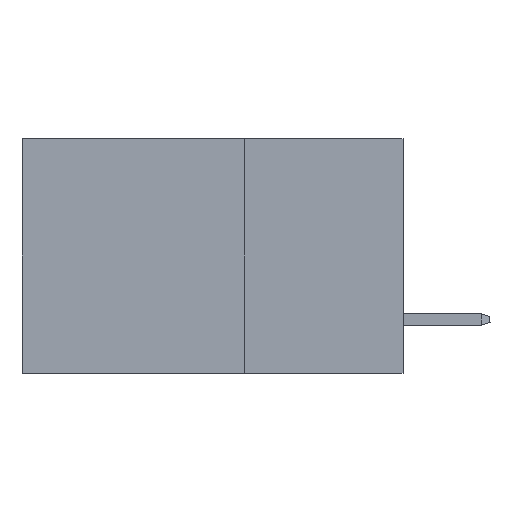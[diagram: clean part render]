
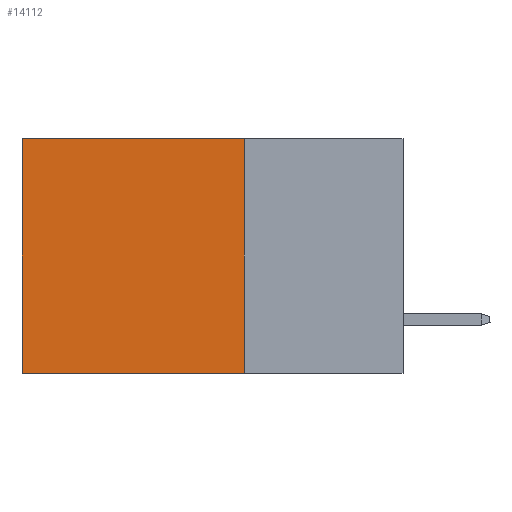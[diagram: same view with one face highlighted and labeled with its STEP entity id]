
A CAD part, left-side view. The second image highlights one B-rep face of the part: STEP entity #14112.
In plain terms, the highlighted planar face has unit normal (-1, 0, 0).
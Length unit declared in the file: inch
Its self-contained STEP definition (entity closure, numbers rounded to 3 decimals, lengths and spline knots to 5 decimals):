
#760 = CARTESIAN_POINT ( 'NONE',  ( 0.2875, 0.25, -0.37 ) ) ;
#1092 = DIRECTION ( 'NONE',  ( 1., 0., 0. ) ) ;
#1314 = CARTESIAN_POINT ( 'NONE',  ( 0.2875, 0.25, 0. ) ) ;
#2424 = VECTOR ( 'NONE', #29652, 39.37008 ) ;
#4251 = LINE ( 'NONE', #760, #14232 ) ;
#4681 = DIRECTION ( 'NONE',  ( 0., 0., -1. ) ) ;
#7620 = DIRECTION ( 'NONE',  ( 0., 0., -1. ) ) ;
#8201 = VERTEX_POINT ( 'NONE', #20159 ) ;
#8949 = ORIENTED_EDGE ( 'NONE', *, *, #25783, .T. ) ;
#11808 = CARTESIAN_POINT ( 'NONE',  ( 0.2875, 0.6, 0. ) ) ;
#12774 = CARTESIAN_POINT ( 'NONE',  ( 0.2875, 0.6, 0. ) ) ;
#12900 = EDGE_CURVE ( 'NONE', #28885, #45731, #36372, .T. ) ;
#14112 = ADVANCED_FACE ( 'NONE', ( #40319 ), #22231, .F. ) ;
#14232 = VECTOR ( 'NONE', #36275, 39.37008 ) ;
#15372 = VERTEX_POINT ( 'NONE', #40328 ) ;
#15742 = LINE ( 'NONE', #11808, #28760 ) ;
#15960 = EDGE_LOOP ( 'NONE', ( #8949, #40078, #38517, #32553 ) ) ;
#16264 = CARTESIAN_POINT ( 'NONE',  ( 0.2875, 0.25, 0. ) ) ;
#20159 = CARTESIAN_POINT ( 'NONE',  ( 0.2875, 0.25, -0.37 ) ) ;
#22231 = PLANE ( 'NONE',  #26239 ) ;
#25783 = EDGE_CURVE ( 'NONE', #45731, #15372, #15742, .T. ) ;
#26239 = AXIS2_PLACEMENT_3D ( 'NONE', #29213, #1092, #7620 ) ;
#28760 = VECTOR ( 'NONE', #44047, 39.37008 ) ;
#28885 = VERTEX_POINT ( 'NONE', #34883 ) ;
#29213 = CARTESIAN_POINT ( 'NONE',  ( 0.2875, 0.25, 0. ) ) ;
#29652 = DIRECTION ( 'NONE',  ( 0., 1., 0. ) ) ;
#31591 = EDGE_CURVE ( 'NONE', #8201, #15372, #4251, .T. ) ;
#32553 = ORIENTED_EDGE ( 'NONE', *, *, #12900, .T. ) ;
#33876 = LINE ( 'NONE', #16264, #42494 ) ;
#34883 = CARTESIAN_POINT ( 'NONE',  ( 0.2875, 0.25, 0. ) ) ;
#36275 = DIRECTION ( 'NONE',  ( 0., 1., 0. ) ) ;
#36372 = LINE ( 'NONE', #1314, #2424 ) ;
#37746 = EDGE_CURVE ( 'NONE', #28885, #8201, #33876, .T. ) ;
#38517 = ORIENTED_EDGE ( 'NONE', *, *, #37746, .F. ) ;
#40078 = ORIENTED_EDGE ( 'NONE', *, *, #31591, .F. ) ;
#40319 = FACE_OUTER_BOUND ( 'NONE', #15960, .T. ) ;
#40328 = CARTESIAN_POINT ( 'NONE',  ( 0.2875, 0.6, -0.37 ) ) ;
#42494 = VECTOR ( 'NONE', #4681, 39.37008 ) ;
#44047 = DIRECTION ( 'NONE',  ( 0., 0., -1. ) ) ;
#45731 = VERTEX_POINT ( 'NONE', #12774 ) ;
